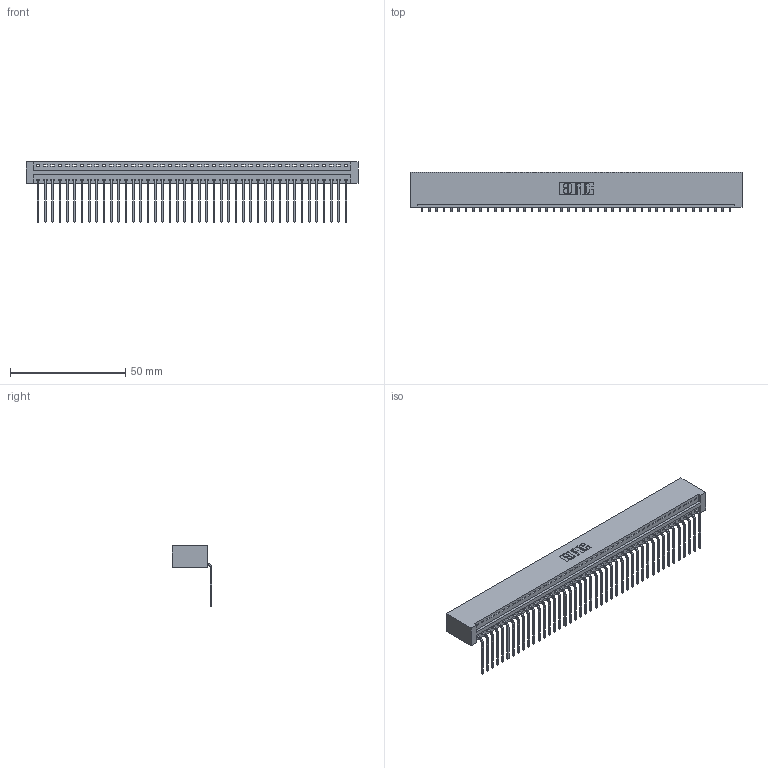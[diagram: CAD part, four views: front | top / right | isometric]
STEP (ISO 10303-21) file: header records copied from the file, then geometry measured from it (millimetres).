
FILE_DESCRIPTION (( 'STEP AP203' ), '1' );
FILE_NAME ('396-043-559-101.STEP', '2019-10-31T23:00:35', ( '' ), ( '' ), 'SwSTEP 2.0', 'SolidWorks 2016', '' );
FILE_SCHEMA (( 'CONFIG_CONTROL_DESIGN' ));
Length unit declared in the file: inch
Products named in the file (3): 346 Part_No Mounting Lugs; 345-292-001_558 559 Tail - 1; 396-043-559-101
Assembly tree (44 placements, depth 2):
  396-043-559-101
    346 Part_No Mounting Lugs
    345-292-001_558 559 Tail - 1  x43
Bounding box: 143.76 x 17.08 x 26.16 mm (x, y, z)
Volume: 14461 mm3; surface area: 19014.9 mm2
Topology: 44 solids, 44 shells, 2694 faces, 8131 edges, 5362 vertices
Faces by surface type: plane 1878, cylinder 816
Entity records: 26359 total; most frequent: CARTESIAN_POINT 4525, ORIENTED_EDGE 4502, DIRECTION 3985, EDGE_CURVE 2251, VECTOR 1955, LINE 1955, VERTEX_POINT 1498, AXIS2_PLACEMENT_3D 1015
